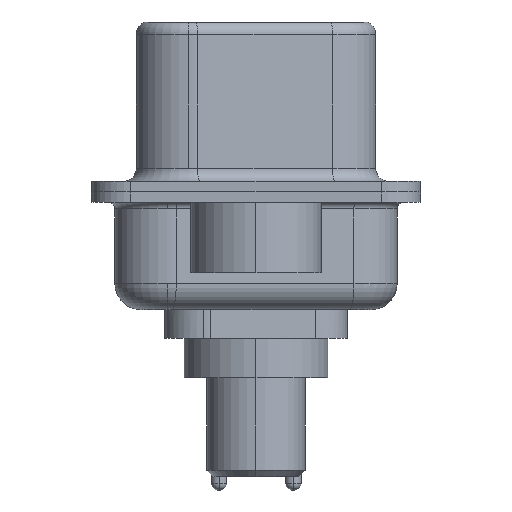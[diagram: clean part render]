
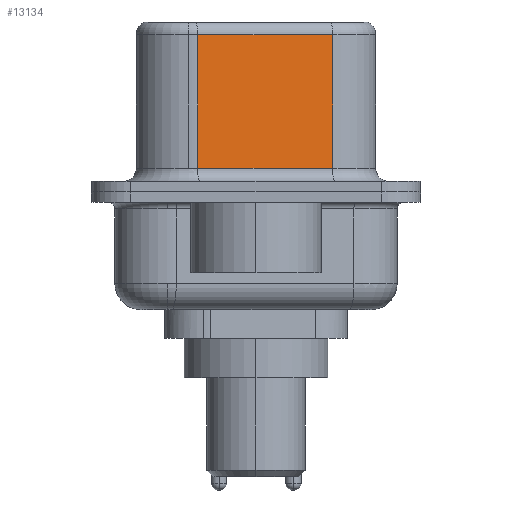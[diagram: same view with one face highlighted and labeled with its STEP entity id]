
A CAD part, left-side view. The second image highlights one B-rep face of the part: STEP entity #13134.
In plain terms, the highlighted planar face has unit normal (-0.985, -0.174, 0).
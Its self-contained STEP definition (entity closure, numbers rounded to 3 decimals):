
#15 = EDGE_LOOP ( 'NONE', ( #5233, #5561, #12461, #112 ) ) ;
#112 = ORIENTED_EDGE ( 'NONE', *, *, #13234, .T. ) ;
#185 = FACE_OUTER_BOUND ( 'NONE', #15, .T. ) ;
#439 = DIRECTION ( 'NONE',  ( 0., 0., -1. ) ) ;
#441 = VECTOR ( 'NONE', #13233, 1000. ) ;
#1528 = DIRECTION ( 'NONE',  ( -0.174, 0.985, 0. ) ) ;
#2167 = LINE ( 'NONE', #14288, #14673 ) ;
#2372 = EDGE_CURVE ( 'NONE', #13580, #5243, #15521, .T. ) ;
#3118 = PLANE ( 'NONE',  #12731 ) ;
#4004 = CARTESIAN_POINT ( 'NONE',  ( 4.565, -2.927, 6.02 ) ) ;
#5233 = ORIENTED_EDGE ( 'NONE', *, *, #14163, .F. ) ;
#5243 = VERTEX_POINT ( 'NONE', #12991 ) ;
#5561 = ORIENTED_EDGE ( 'NONE', *, *, #2372, .T. ) ;
#6563 = VERTEX_POINT ( 'NONE', #10771 ) ;
#6637 = LINE ( 'NONE', #9564, #441 ) ;
#6740 = DIRECTION ( 'NONE',  ( 0.985, 0.174, 0. ) ) ;
#6899 = DIRECTION ( 'NONE',  ( 0.174, -0.985, 0. ) ) ;
#6933 = CARTESIAN_POINT ( 'NONE',  ( 4.565, -2.927, 6.02 ) ) ;
#8676 = EDGE_CURVE ( 'NONE', #5243, #12008, #6637, .T. ) ;
#9391 = CARTESIAN_POINT ( 'NONE',  ( 3.655, 2.233, 0.9 ) ) ;
#9564 = CARTESIAN_POINT ( 'NONE',  ( 3.655, 2.233, 6.52 ) ) ;
#9650 = VECTOR ( 'NONE', #439, 1000. ) ;
#9985 = CARTESIAN_POINT ( 'NONE',  ( 4.565, -2.927, 6.52 ) ) ;
#10771 = CARTESIAN_POINT ( 'NONE',  ( 4.565, -2.927, 0.9 ) ) ;
#12008 = VERTEX_POINT ( 'NONE', #9391 ) ;
#12194 = VECTOR ( 'NONE', #1528, 1000. ) ;
#12461 = ORIENTED_EDGE ( 'NONE', *, *, #8676, .T. ) ;
#12731 = AXIS2_PLACEMENT_3D ( 'NONE', #14131, #6740, #15399 ) ;
#12991 = CARTESIAN_POINT ( 'NONE',  ( 3.655, 2.233, 6.02 ) ) ;
#13134 = ADVANCED_FACE ( 'NONE', ( #185 ), #3118, .F. ) ;
#13233 = DIRECTION ( 'NONE',  ( 0., 0., -1. ) ) ;
#13234 = EDGE_CURVE ( 'NONE', #12008, #6563, #2167, .T. ) ;
#13271 = LINE ( 'NONE', #9985, #9650 ) ;
#13580 = VERTEX_POINT ( 'NONE', #4004 ) ;
#14131 = CARTESIAN_POINT ( 'NONE',  ( 4.565, -2.927, 6.52 ) ) ;
#14163 = EDGE_CURVE ( 'NONE', #13580, #6563, #13271, .T. ) ;
#14288 = CARTESIAN_POINT ( 'NONE',  ( 4.565, -2.927, 0.9 ) ) ;
#14673 = VECTOR ( 'NONE', #6899, 1000. ) ;
#15399 = DIRECTION ( 'NONE',  ( -0.174, 0.985, 0. ) ) ;
#15521 = LINE ( 'NONE', #6933, #12194 ) ;
